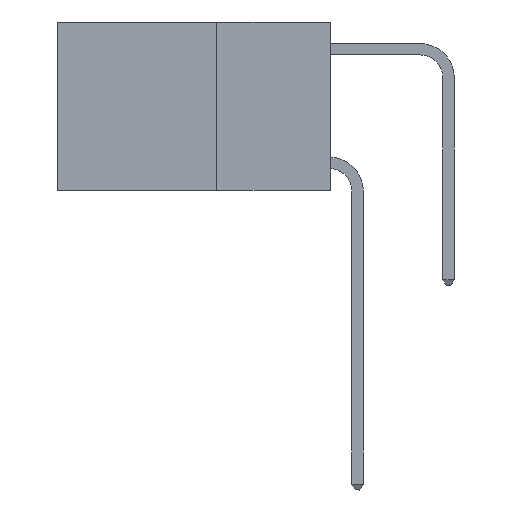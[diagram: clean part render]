
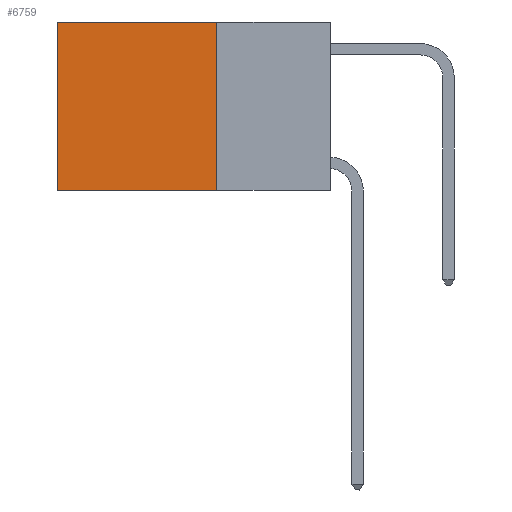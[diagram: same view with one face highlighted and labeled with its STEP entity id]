
A CAD part, left-side view. The second image highlights one B-rep face of the part: STEP entity #6759.
In plain terms, the highlighted planar face has unit normal (-1, 0, 0).
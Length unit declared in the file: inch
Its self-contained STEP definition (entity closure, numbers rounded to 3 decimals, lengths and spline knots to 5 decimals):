
#519 = VECTOR ( 'NONE', #8577, 39.37008 ) ;
#1780 = DIRECTION ( 'NONE',  ( 0., 1., 0. ) ) ;
#2191 = CARTESIAN_POINT ( 'NONE',  ( 0.2625, 0.6, -0.37 ) ) ;
#2684 = ORIENTED_EDGE ( 'NONE', *, *, #18570, .T. ) ;
#3694 = CARTESIAN_POINT ( 'NONE',  ( 0.2625, 0.6, 0. ) ) ;
#4341 = CARTESIAN_POINT ( 'NONE',  ( 0.2625, 0.25, 0. ) ) ;
#5726 = ORIENTED_EDGE ( 'NONE', *, *, #13945, .T. ) ;
#6013 = CARTESIAN_POINT ( 'NONE',  ( 0.2625, 0.25, 0. ) ) ;
#6253 = LINE ( 'NONE', #6665, #519 ) ;
#6263 = DIRECTION ( 'NONE',  ( 0., 0., -1. ) ) ;
#6418 = CARTESIAN_POINT ( 'NONE',  ( 0.2625, 0.6, 0. ) ) ;
#6665 = CARTESIAN_POINT ( 'NONE',  ( 0.2625, 0.25, 0. ) ) ;
#6759 = ADVANCED_FACE ( 'NONE', ( #10445 ), #15711, .F. ) ;
#7732 = VERTEX_POINT ( 'NONE', #8968 ) ;
#8577 = DIRECTION ( 'NONE',  ( 0., 0., -1. ) ) ;
#8616 = DIRECTION ( 'NONE',  ( 0., 1., 0. ) ) ;
#8968 = CARTESIAN_POINT ( 'NONE',  ( 0.2625, 0.25, -0.37 ) ) ;
#9023 = VECTOR ( 'NONE', #23512, 39.37008 ) ;
#9771 = VERTEX_POINT ( 'NONE', #6013 ) ;
#9969 = EDGE_LOOP ( 'NONE', ( #5726, #12729, #20492, #2684 ) ) ;
#10445 = FACE_OUTER_BOUND ( 'NONE', #9969, .T. ) ;
#10678 = VECTOR ( 'NONE', #1780, 39.37008 ) ;
#11335 = CARTESIAN_POINT ( 'NONE',  ( 0.2625, 0.25, 0. ) ) ;
#12044 = LINE ( 'NONE', #21804, #12653 ) ;
#12653 = VECTOR ( 'NONE', #8616, 39.37008 ) ;
#12729 = ORIENTED_EDGE ( 'NONE', *, *, #13328, .F. ) ;
#13328 = EDGE_CURVE ( 'NONE', #7732, #17679, #12044, .T. ) ;
#13945 = EDGE_CURVE ( 'NONE', #24305, #17679, #14095, .T. ) ;
#14095 = LINE ( 'NONE', #6418, #9023 ) ;
#15672 = LINE ( 'NONE', #11335, #10678 ) ;
#15711 = PLANE ( 'NONE',  #24281 ) ;
#17218 = EDGE_CURVE ( 'NONE', #9771, #7732, #6253, .T. ) ;
#17584 = DIRECTION ( 'NONE',  ( 1., 0., 0. ) ) ;
#17679 = VERTEX_POINT ( 'NONE', #2191 ) ;
#18570 = EDGE_CURVE ( 'NONE', #9771, #24305, #15672, .T. ) ;
#20492 = ORIENTED_EDGE ( 'NONE', *, *, #17218, .F. ) ;
#21804 = CARTESIAN_POINT ( 'NONE',  ( 0.2625, 0.25, -0.37 ) ) ;
#23512 = DIRECTION ( 'NONE',  ( 0., 0., -1. ) ) ;
#24281 = AXIS2_PLACEMENT_3D ( 'NONE', #4341, #17584, #6263 ) ;
#24305 = VERTEX_POINT ( 'NONE', #3694 ) ;
